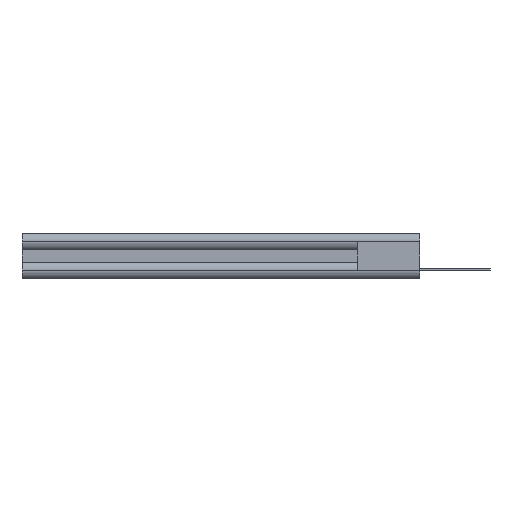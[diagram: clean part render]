
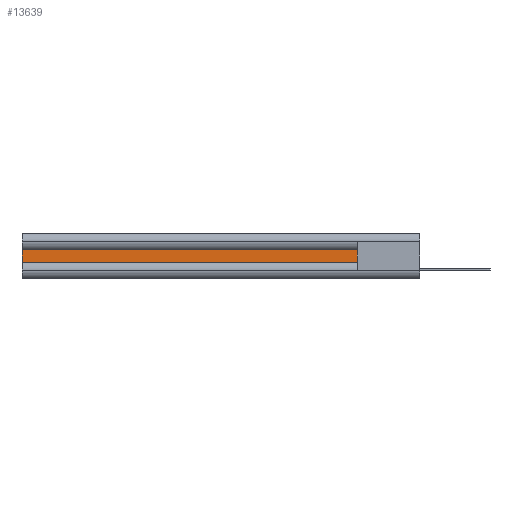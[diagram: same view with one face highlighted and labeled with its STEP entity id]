
A CAD part, left-side view. The second image highlights one B-rep face of the part: STEP entity #13639.
In plain terms, the highlighted planar face has unit normal (-1, 0, 0).
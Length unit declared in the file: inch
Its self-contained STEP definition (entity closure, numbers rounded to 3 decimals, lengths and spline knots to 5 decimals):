
#75 = DIRECTION ( 'NONE',  ( 0., 1., 0. ) ) ;
#408 = DIRECTION ( 'NONE',  ( 0., 0., -1. ) ) ;
#1299 = VERTEX_POINT ( 'NONE', #17890 ) ;
#1912 = LINE ( 'NONE', #10780, #6494 ) ;
#3171 = CARTESIAN_POINT ( 'NONE',  ( 0.044, 0.37012, -0.0465 ) ) ;
#3878 = ORIENTED_EDGE ( 'NONE', *, *, #19949, .T. ) ;
#4917 = DIRECTION ( 'NONE',  ( 1., 0., 0. ) ) ;
#5155 = VECTOR ( 'NONE', #14610, 39.37008 ) ;
#5862 = VERTEX_POINT ( 'NONE', #10376 ) ;
#6314 = VERTEX_POINT ( 'NONE', #13336 ) ;
#6494 = VECTOR ( 'NONE', #408, 39.37008 ) ;
#7672 = ORIENTED_EDGE ( 'NONE', *, *, #10877, .F. ) ;
#7739 = CARTESIAN_POINT ( 'NONE',  ( 0.044, 0.37012, 0.0465 ) ) ;
#10376 = CARTESIAN_POINT ( 'NONE',  ( 0.044, 3., -0.0465 ) ) ;
#10780 = CARTESIAN_POINT ( 'NONE',  ( 0.044, 0.473, -0.0465 ) ) ;
#10877 = EDGE_CURVE ( 'NONE', #1299, #17979, #1912, .T. ) ;
#11248 = VECTOR ( 'NONE', #13043, 39.37008 ) ;
#11325 = CARTESIAN_POINT ( 'NONE',  ( 0.044, 3., -0.0465 ) ) ;
#12168 = AXIS2_PLACEMENT_3D ( 'NONE', #3171, #4917, #16872 ) ;
#13043 = DIRECTION ( 'NONE',  ( 0., 0., -1. ) ) ;
#13336 = CARTESIAN_POINT ( 'NONE',  ( 0.044, 3., 0.0465 ) ) ;
#13381 = CARTESIAN_POINT ( 'NONE',  ( 0.044, 0.473, -0.0465 ) ) ;
#13467 = PLANE ( 'NONE',  #12168 ) ;
#13505 = EDGE_LOOP ( 'NONE', ( #13763, #3878, #13593, #7672 ) ) ;
#13593 = ORIENTED_EDGE ( 'NONE', *, *, #20886, .F. ) ;
#13639 = ADVANCED_FACE ( 'NONE', ( #17353 ), #13467, .F. ) ;
#13763 = ORIENTED_EDGE ( 'NONE', *, *, #18449, .T. ) ;
#14252 = LINE ( 'NONE', #7739, #5155 ) ;
#14610 = DIRECTION ( 'NONE',  ( 0., 1., 0. ) ) ;
#15772 = LINE ( 'NONE', #11325, #11248 ) ;
#16872 = DIRECTION ( 'NONE',  ( 0., 0., -1. ) ) ;
#17045 = VECTOR ( 'NONE', #75, 39.37008 ) ;
#17353 = FACE_OUTER_BOUND ( 'NONE', #13505, .T. ) ;
#17576 = LINE ( 'NONE', #19427, #17045 ) ;
#17890 = CARTESIAN_POINT ( 'NONE',  ( 0.044, 0.473, 0.0465 ) ) ;
#17979 = VERTEX_POINT ( 'NONE', #13381 ) ;
#18449 = EDGE_CURVE ( 'NONE', #1299, #6314, #14252, .T. ) ;
#19427 = CARTESIAN_POINT ( 'NONE',  ( 0.044, 0.37012, -0.0465 ) ) ;
#19949 = EDGE_CURVE ( 'NONE', #6314, #5862, #15772, .T. ) ;
#20886 = EDGE_CURVE ( 'NONE', #17979, #5862, #17576, .T. ) ;
